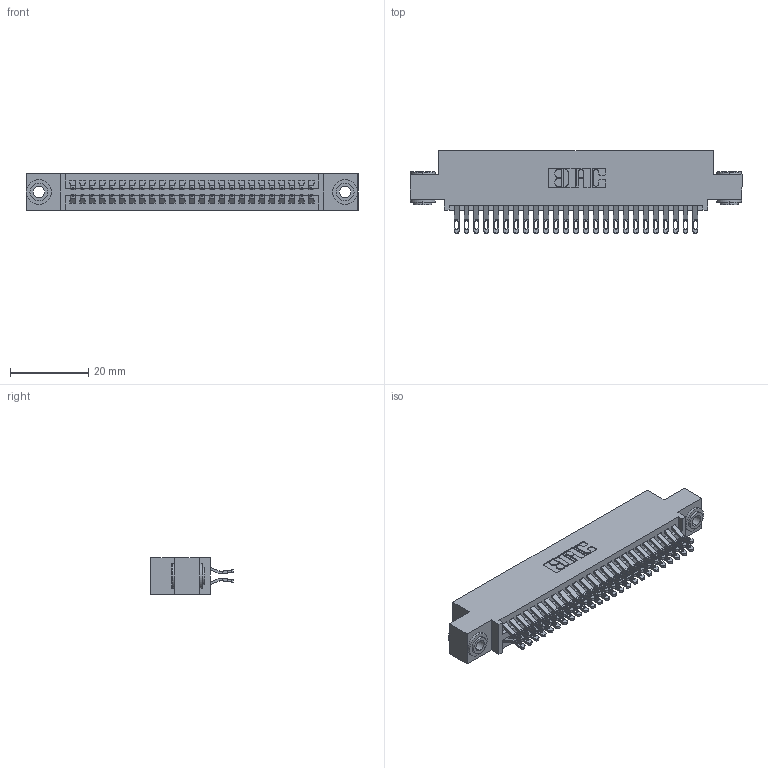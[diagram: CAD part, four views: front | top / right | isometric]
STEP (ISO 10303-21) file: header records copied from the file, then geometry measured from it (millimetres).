
FILE_DESCRIPTION (( 'STEP AP203' ), '1' );
FILE_NAME ('395-050-555-503.STEP', '2018-11-20T09:50:26', ( '' ), ( '' ), 'SwSTEP 2.0', 'SolidWorks 2016', '' );
FILE_SCHEMA (( 'CONFIG_CONTROL_DESIGN' ));
Length unit declared in the file: inch
Products named in the file (4): 345 Part_0.110 Offset - 0.156 Dia-TH; 345-292-001_555 Tail; 395-050-555-503; 345-250-002_345-250-002-102
Assembly tree (53 placements, depth 2):
  395-050-555-503
    345 Part_0.110 Offset - 0.156 Dia-TH
    345-292-001_555 Tail  x50
    345-250-002_345-250-002-102  x2
Bounding box: 84.71 x 21.13 x 9.4 mm (x, y, z)
Volume: 8162 mm3; surface area: 12537.7 mm2
Topology: 53 solids, 53 shells, 2968 faces, 9279 edges, 6182 vertices
Faces by surface type: plane 1644, cylinder 1316, cone 8
Entity records: 23012 total; most frequent: CARTESIAN_POINT 3885, ORIENTED_EDGE 3782, DIRECTION 3445, EDGE_CURVE 1891, LINE 1615, VECTOR 1615, VERTEX_POINT 1258, AXIS2_PLACEMENT_3D 915
